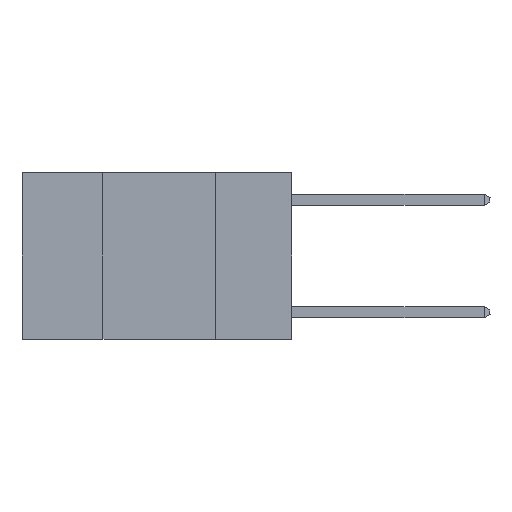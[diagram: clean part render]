
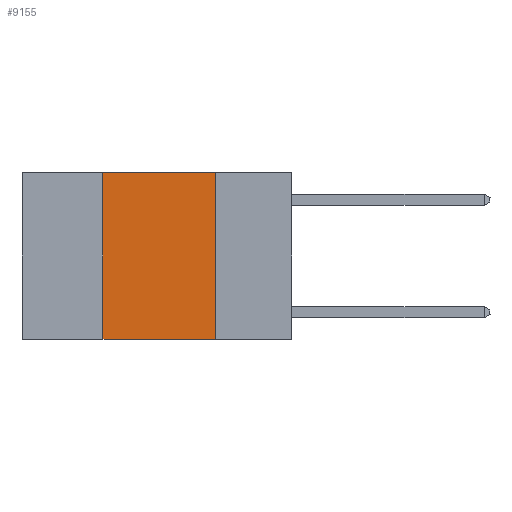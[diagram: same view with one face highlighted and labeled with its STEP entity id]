
A CAD part, left-side view. The second image highlights one B-rep face of the part: STEP entity #9155.
In plain terms, the highlighted planar face has unit normal (-1, 0, 0).
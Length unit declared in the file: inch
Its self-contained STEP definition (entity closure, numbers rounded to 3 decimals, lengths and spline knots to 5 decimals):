
#44 = VECTOR ( 'NONE', #557, 39.37008 ) ;
#265 = DIRECTION ( 'NONE',  ( 0., 0., -1. ) ) ;
#357 = CARTESIAN_POINT ( 'NONE',  ( 0., 0.42, 0. ) ) ;
#557 = DIRECTION ( 'NONE',  ( 0., -1., 0. ) ) ;
#1286 = LINE ( 'NONE', #8483, #3207 ) ;
#1528 = LINE ( 'NONE', #5807, #44 ) ;
#1613 = EDGE_CURVE ( 'NONE', #9840, #5331, #5686, .T. ) ;
#2644 = EDGE_CURVE ( 'NONE', #9865, #5331, #1286, .T. ) ;
#2774 = CARTESIAN_POINT ( 'NONE',  ( 0., 0.17, -0.37 ) ) ;
#3207 = VECTOR ( 'NONE', #9429, 39.37008 ) ;
#3518 = EDGE_CURVE ( 'NONE', #9947, #9865, #1528, .T. ) ;
#3525 = ORIENTED_EDGE ( 'NONE', *, *, #1613, .T. ) ;
#4557 = CARTESIAN_POINT ( 'NONE',  ( 0., 0.17, 0. ) ) ;
#4580 = CARTESIAN_POINT ( 'NONE',  ( 0., 0.6, 0. ) ) ;
#4652 = LINE ( 'NONE', #9159, #7480 ) ;
#4799 = FACE_OUTER_BOUND ( 'NONE', #7714, .T. ) ;
#5119 = AXIS2_PLACEMENT_3D ( 'NONE', #4580, #5553, #265 ) ;
#5331 = VERTEX_POINT ( 'NONE', #2774 ) ;
#5498 = PLANE ( 'NONE',  #5119 ) ;
#5553 = DIRECTION ( 'NONE',  ( 1., 0., 0. ) ) ;
#5686 = LINE ( 'NONE', #5743, #11303 ) ;
#5743 = CARTESIAN_POINT ( 'NONE',  ( 0., 0.6, -0.37 ) ) ;
#5807 = CARTESIAN_POINT ( 'NONE',  ( 0., 0.6, 0. ) ) ;
#6175 = CARTESIAN_POINT ( 'NONE',  ( 0., 0.42, -0.37 ) ) ;
#6458 = DIRECTION ( 'NONE',  ( 0., 0., 1. ) ) ;
#6885 = EDGE_CURVE ( 'NONE', #9840, #9947, #4652, .T. ) ;
#7480 = VECTOR ( 'NONE', #6458, 39.37008 ) ;
#7695 = ORIENTED_EDGE ( 'NONE', *, *, #2644, .F. ) ;
#7714 = EDGE_LOOP ( 'NONE', ( #7695, #8060, #8958, #3525 ) ) ;
#8060 = ORIENTED_EDGE ( 'NONE', *, *, #3518, .F. ) ;
#8483 = CARTESIAN_POINT ( 'NONE',  ( 0., 0.17, 0. ) ) ;
#8958 = ORIENTED_EDGE ( 'NONE', *, *, #6885, .F. ) ;
#9155 = ADVANCED_FACE ( 'NONE', ( #4799 ), #5498, .F. ) ;
#9159 = CARTESIAN_POINT ( 'NONE',  ( 0., 0.42, 0. ) ) ;
#9429 = DIRECTION ( 'NONE',  ( 0., 0., -1. ) ) ;
#9840 = VERTEX_POINT ( 'NONE', #6175 ) ;
#9865 = VERTEX_POINT ( 'NONE', #4557 ) ;
#9947 = VERTEX_POINT ( 'NONE', #357 ) ;
#10188 = DIRECTION ( 'NONE',  ( 0., -1., 0. ) ) ;
#11303 = VECTOR ( 'NONE', #10188, 39.37008 ) ;
